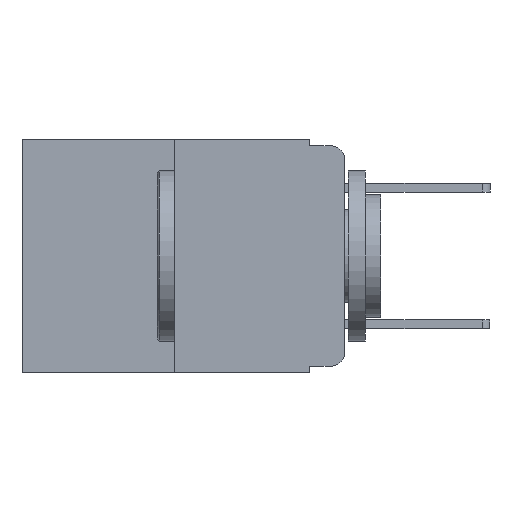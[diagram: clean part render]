
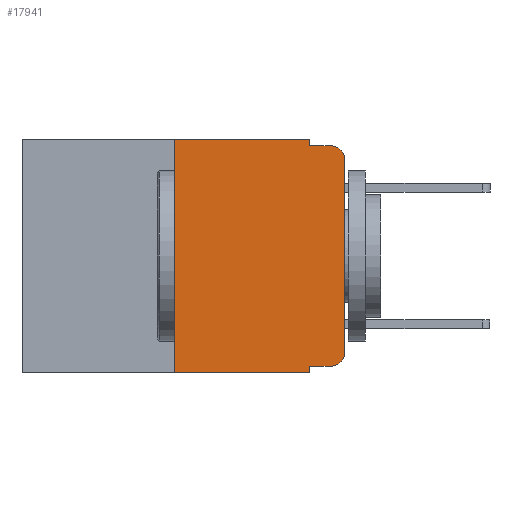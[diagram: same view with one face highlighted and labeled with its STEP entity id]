
A CAD part, left-side view. The second image highlights one B-rep face of the part: STEP entity #17941.
In plain terms, the highlighted planar face has unit normal (-1, 0, 0).
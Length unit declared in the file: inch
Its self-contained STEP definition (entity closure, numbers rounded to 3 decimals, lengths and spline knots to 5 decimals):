
#31 = VERTEX_POINT ( 'NONE', #15982 ) ;
#32 = ORIENTED_EDGE ( 'NONE', *, *, #19920, .F. ) ;
#39 = VERTEX_POINT ( 'NONE', #19868 ) ;
#124 = CARTESIAN_POINT ( 'NONE',  ( 0., 0.25, 0. ) ) ;
#340 = CARTESIAN_POINT ( 'NONE',  ( 0., 0.473, 0. ) ) ;
#465 = ORIENTED_EDGE ( 'NONE', *, *, #15330, .T. ) ;
#639 = ORIENTED_EDGE ( 'NONE', *, *, #1327, .F. ) ;
#932 = ORIENTED_EDGE ( 'NONE', *, *, #16529, .T. ) ;
#1327 = EDGE_CURVE ( 'NONE', #17160, #5915, #16647, .T. ) ;
#1409 = ORIENTED_EDGE ( 'NONE', *, *, #17312, .T. ) ;
#1668 = CARTESIAN_POINT ( 'NONE',  ( 0., 0.051, -0.01 ) ) ;
#1929 = DIRECTION ( 'NONE',  ( 0., -1., 0. ) ) ;
#2016 = VECTOR ( 'NONE', #18895, 39.37008 ) ;
#2293 = DIRECTION ( 'NONE',  ( 1., 0., 0. ) ) ;
#2637 = LINE ( 'NONE', #13297, #2016 ) ;
#2696 = LINE ( 'NONE', #5857, #7175 ) ;
#2804 = ORIENTED_EDGE ( 'NONE', *, *, #3403, .T. ) ;
#3403 = EDGE_CURVE ( 'NONE', #12216, #7130, #21998, .T. ) ;
#3531 = CARTESIAN_POINT ( 'NONE',  ( 0., 0., 0. ) ) ;
#3600 = LINE ( 'NONE', #1668, #7482 ) ;
#3623 = CARTESIAN_POINT ( 'NONE',  ( 0., 0., -0.03 ) ) ;
#3862 = CARTESIAN_POINT ( 'NONE',  ( 0., 0.25, -0.343 ) ) ;
#4082 = EDGE_CURVE ( 'NONE', #39, #21393, #3600, .T. ) ;
#4181 = DIRECTION ( 'NONE',  ( 0., -1., 0. ) ) ;
#4306 = ORIENTED_EDGE ( 'NONE', *, *, #22169, .T. ) ;
#4407 = CIRCLE ( 'NONE', #9803, 0.02 ) ;
#5857 = CARTESIAN_POINT ( 'NONE',  ( 0., 0.473, 0. ) ) ;
#5915 = VERTEX_POINT ( 'NONE', #7521 ) ;
#6052 = AXIS2_PLACEMENT_3D ( 'NONE', #8724, #21676, #10617 ) ;
#6946 = ORIENTED_EDGE ( 'NONE', *, *, #4082, .F. ) ;
#7130 = VERTEX_POINT ( 'NONE', #3623 ) ;
#7175 = VECTOR ( 'NONE', #22442, 39.37008 ) ;
#7441 = CARTESIAN_POINT ( 'NONE',  ( 0., 0.051, -0.333 ) ) ;
#7482 = VECTOR ( 'NONE', #1929, 39.37008 ) ;
#7521 = CARTESIAN_POINT ( 'NONE',  ( 0., 0.051, -0.343 ) ) ;
#7778 = DIRECTION ( 'NONE',  ( 0., 0., 1. ) ) ;
#8012 = CARTESIAN_POINT ( 'NONE',  ( 0., 0.02, -0.313 ) ) ;
#8605 = CARTESIAN_POINT ( 'NONE',  ( 0., 0.051, 0. ) ) ;
#8724 = CARTESIAN_POINT ( 'NONE',  ( 0., 0.02, -0.03 ) ) ;
#8821 = DIRECTION ( 'NONE',  ( 0., 0., -1. ) ) ;
#9610 = ORIENTED_EDGE ( 'NONE', *, *, #15440, .F. ) ;
#9803 = AXIS2_PLACEMENT_3D ( 'NONE', #8012, #20993, #9898 ) ;
#9892 = CARTESIAN_POINT ( 'NONE',  ( 0., 0.473, -0.343 ) ) ;
#9898 = DIRECTION ( 'NONE',  ( 0., 0., -1. ) ) ;
#10040 = CIRCLE ( 'NONE', #6052, 0.02 ) ;
#10256 = CARTESIAN_POINT ( 'NONE',  ( 0., 0.02, -0.01 ) ) ;
#10617 = DIRECTION ( 'NONE',  ( 0., 0., -1. ) ) ;
#10792 = ORIENTED_EDGE ( 'NONE', *, *, #19914, .F. ) ;
#11098 = VECTOR ( 'NONE', #8821, 39.37008 ) ;
#12193 = LINE ( 'NONE', #124, #21401 ) ;
#12216 = VERTEX_POINT ( 'NONE', #16161 ) ;
#12248 = VERTEX_POINT ( 'NONE', #18088 ) ;
#12605 = CARTESIAN_POINT ( 'NONE',  ( 0., 0.02, -0.333 ) ) ;
#13297 = CARTESIAN_POINT ( 'NONE',  ( 0., 0.051, -0.333 ) ) ;
#13905 = LINE ( 'NONE', #9892, #18841 ) ;
#15222 = VERTEX_POINT ( 'NONE', #3862 ) ;
#15330 = EDGE_CURVE ( 'NONE', #15222, #5915, #13905, .T. ) ;
#15362 = VECTOR ( 'NONE', #15857, 39.37008 ) ;
#15440 = EDGE_CURVE ( 'NONE', #31, #39, #15936, .T. ) ;
#15517 = DIRECTION ( 'NONE',  ( 0., 0., -1. ) ) ;
#15777 = CARTESIAN_POINT ( 'NONE',  ( 0., 0.051, 0. ) ) ;
#15857 = DIRECTION ( 'NONE',  ( 0., 0., -1. ) ) ;
#15936 = LINE ( 'NONE', #15777, #15362 ) ;
#15982 = CARTESIAN_POINT ( 'NONE',  ( 0., 0.051, 0. ) ) ;
#16071 = EDGE_LOOP ( 'NONE', ( #2804, #4306, #6946, #9610, #10792, #32, #465, #639, #932, #1409 ) ) ;
#16161 = CARTESIAN_POINT ( 'NONE',  ( 0., 0., -0.313 ) ) ;
#16529 = EDGE_CURVE ( 'NONE', #17160, #20310, #2637, .T. ) ;
#16647 = LINE ( 'NONE', #8605, #11098 ) ;
#17160 = VERTEX_POINT ( 'NONE', #7441 ) ;
#17312 = EDGE_CURVE ( 'NONE', #20310, #12216, #4407, .T. ) ;
#17381 = DIRECTION ( 'NONE',  ( 0., 0., 1. ) ) ;
#17941 = ADVANCED_FACE ( 'NONE', ( #22380 ), #22785, .F. ) ;
#18088 = CARTESIAN_POINT ( 'NONE',  ( 0., 0.25, 0. ) ) ;
#18841 = VECTOR ( 'NONE', #4181, 39.37008 ) ;
#18895 = DIRECTION ( 'NONE',  ( 0., -1., 0. ) ) ;
#19868 = CARTESIAN_POINT ( 'NONE',  ( 0., 0.051, -0.01 ) ) ;
#19914 = EDGE_CURVE ( 'NONE', #12248, #31, #2696, .T. ) ;
#19920 = EDGE_CURVE ( 'NONE', #15222, #12248, #12193, .T. ) ;
#20310 = VERTEX_POINT ( 'NONE', #12605 ) ;
#20880 = VECTOR ( 'NONE', #17381, 39.37008 ) ;
#20993 = DIRECTION ( 'NONE',  ( -1., 0., 0. ) ) ;
#21286 = AXIS2_PLACEMENT_3D ( 'NONE', #340, #2293, #15517 ) ;
#21393 = VERTEX_POINT ( 'NONE', #10256 ) ;
#21401 = VECTOR ( 'NONE', #7778, 39.37008 ) ;
#21676 = DIRECTION ( 'NONE',  ( -1., 0., 0. ) ) ;
#21998 = LINE ( 'NONE', #3531, #20880 ) ;
#22169 = EDGE_CURVE ( 'NONE', #7130, #21393, #10040, .T. ) ;
#22380 = FACE_OUTER_BOUND ( 'NONE', #16071, .T. ) ;
#22442 = DIRECTION ( 'NONE',  ( 0., -1., 0. ) ) ;
#22785 = PLANE ( 'NONE',  #21286 ) ;
